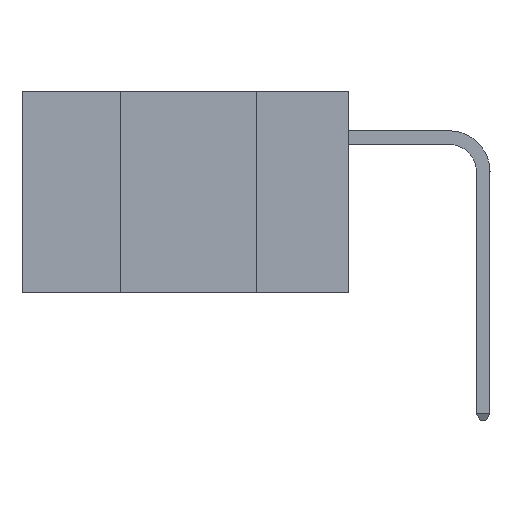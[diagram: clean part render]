
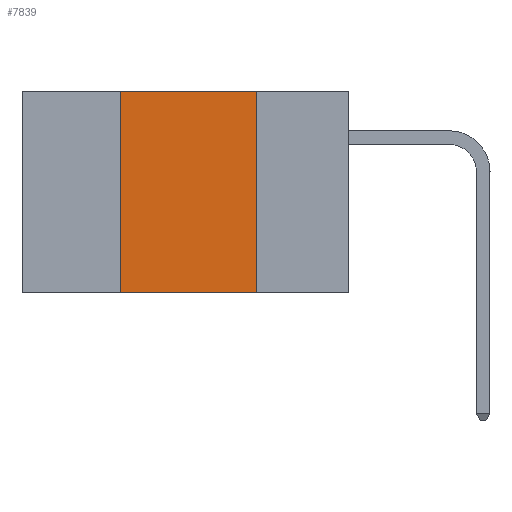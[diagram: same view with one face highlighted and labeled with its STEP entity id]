
A CAD part, left-side view. The second image highlights one B-rep face of the part: STEP entity #7839.
In plain terms, the highlighted planar face has unit normal (-1, 0, 0).
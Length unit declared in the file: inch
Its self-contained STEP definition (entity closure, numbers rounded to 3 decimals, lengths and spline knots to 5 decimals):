
#416 = ORIENTED_EDGE ( 'NONE', *, *, #7066, .F. ) ;
#941 = VECTOR ( 'NONE', #17131, 39.37008 ) ;
#1111 = VERTEX_POINT ( 'NONE', #10308 ) ;
#1257 = ORIENTED_EDGE ( 'NONE', *, *, #4351, .T. ) ;
#1899 = ORIENTED_EDGE ( 'NONE', *, *, #16170, .F. ) ;
#3035 = DIRECTION ( 'NONE',  ( 0., -1., 0. ) ) ;
#3564 = CARTESIAN_POINT ( 'NONE',  ( 0., 0.42, 0. ) ) ;
#4351 = EDGE_CURVE ( 'NONE', #8209, #1111, #13122, .T. ) ;
#4641 = CARTESIAN_POINT ( 'NONE',  ( 0., 0.42, -0.37 ) ) ;
#5193 = PLANE ( 'NONE',  #7624 ) ;
#6122 = VECTOR ( 'NONE', #3035, 39.37008 ) ;
#6541 = DIRECTION ( 'NONE',  ( 1., 0., 0. ) ) ;
#7066 = EDGE_CURVE ( 'NONE', #8209, #12573, #12234, .T. ) ;
#7106 = LINE ( 'NONE', #8777, #8372 ) ;
#7624 = AXIS2_PLACEMENT_3D ( 'NONE', #14713, #6541, #16056 ) ;
#7839 = ADVANCED_FACE ( 'NONE', ( #9239 ), #5193, .F. ) ;
#7977 = VERTEX_POINT ( 'NONE', #16340 ) ;
#8209 = VERTEX_POINT ( 'NONE', #4641 ) ;
#8372 = VECTOR ( 'NONE', #16907, 39.37008 ) ;
#8410 = CARTESIAN_POINT ( 'NONE',  ( 0., 0.6, 0. ) ) ;
#8777 = CARTESIAN_POINT ( 'NONE',  ( 0., 0.17, 0. ) ) ;
#9063 = VECTOR ( 'NONE', #13985, 39.37008 ) ;
#9239 = FACE_OUTER_BOUND ( 'NONE', #12151, .T. ) ;
#9988 = ORIENTED_EDGE ( 'NONE', *, *, #12842, .F. ) ;
#10308 = CARTESIAN_POINT ( 'NONE',  ( 0., 0.17, -0.37 ) ) ;
#12151 = EDGE_LOOP ( 'NONE', ( #1899, #9988, #416, #1257 ) ) ;
#12234 = LINE ( 'NONE', #3564, #941 ) ;
#12551 = CARTESIAN_POINT ( 'NONE',  ( 0., 0.6, -0.37 ) ) ;
#12573 = VERTEX_POINT ( 'NONE', #16982 ) ;
#12842 = EDGE_CURVE ( 'NONE', #12573, #7977, #16517, .T. ) ;
#13122 = LINE ( 'NONE', #12551, #9063 ) ;
#13985 = DIRECTION ( 'NONE',  ( 0., -1., 0. ) ) ;
#14713 = CARTESIAN_POINT ( 'NONE',  ( 0., 0.6, 0. ) ) ;
#16056 = DIRECTION ( 'NONE',  ( 0., 0., -1. ) ) ;
#16170 = EDGE_CURVE ( 'NONE', #7977, #1111, #7106, .T. ) ;
#16340 = CARTESIAN_POINT ( 'NONE',  ( 0., 0.17, 0. ) ) ;
#16517 = LINE ( 'NONE', #8410, #6122 ) ;
#16907 = DIRECTION ( 'NONE',  ( 0., 0., -1. ) ) ;
#16982 = CARTESIAN_POINT ( 'NONE',  ( 0., 0.42, 0. ) ) ;
#17131 = DIRECTION ( 'NONE',  ( 0., 0., 1. ) ) ;
